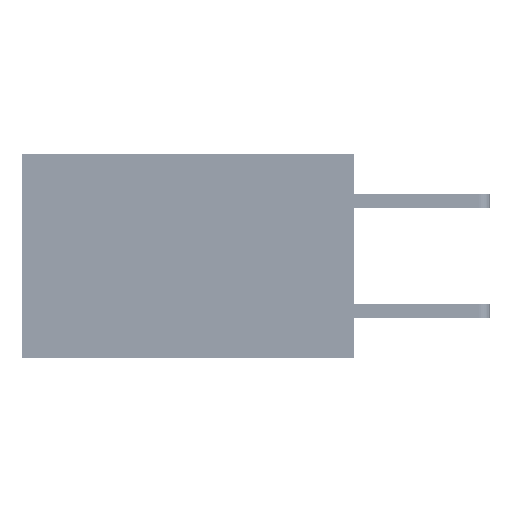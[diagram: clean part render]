
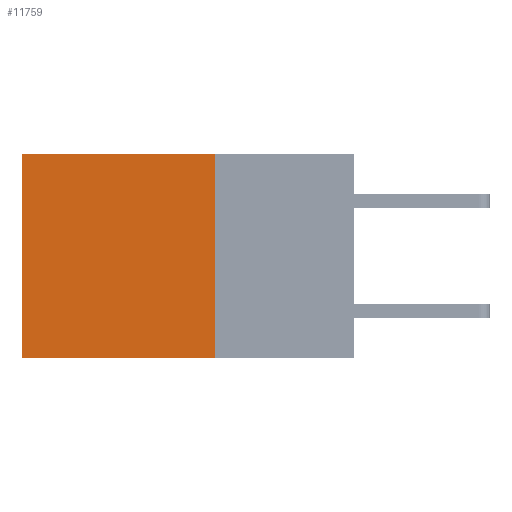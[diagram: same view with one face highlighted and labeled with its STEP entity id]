
A CAD part, left-side view. The second image highlights one B-rep face of the part: STEP entity #11759.
In plain terms, the highlighted planar face has unit normal (-1, 0, 0).
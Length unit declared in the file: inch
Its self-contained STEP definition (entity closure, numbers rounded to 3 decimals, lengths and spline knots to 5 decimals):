
#631 = DIRECTION ( 'NONE',  ( 0., 0., -1. ) ) ;
#2991 = VERTEX_POINT ( 'NONE', #26524 ) ;
#5545 = PLANE ( 'NONE',  #13367 ) ;
#6780 = LINE ( 'NONE', #41627, #39125 ) ;
#8586 = DIRECTION ( 'NONE',  ( 0., 0., -1. ) ) ;
#9468 = EDGE_CURVE ( 'NONE', #12909, #18401, #6780, .T. ) ;
#11207 = CARTESIAN_POINT ( 'NONE',  ( 0.2875, 0.25, 0. ) ) ;
#11418 = LINE ( 'NONE', #24090, #28578 ) ;
#11658 = CARTESIAN_POINT ( 'NONE',  ( 0.2875, 0.25, 0. ) ) ;
#11759 = ADVANCED_FACE ( 'NONE', ( #35280 ), #5545, .F. ) ;
#12386 = EDGE_LOOP ( 'NONE', ( #23890, #41944, #21799, #23471 ) ) ;
#12909 = VERTEX_POINT ( 'NONE', #42893 ) ;
#13367 = AXIS2_PLACEMENT_3D ( 'NONE', #28836, #28555, #8586 ) ;
#13528 = VECTOR ( 'NONE', #28085, 39.37008 ) ;
#18401 = VERTEX_POINT ( 'NONE', #35688 ) ;
#19248 = CARTESIAN_POINT ( 'NONE',  ( 0.2875, 0.25, 0. ) ) ;
#19585 = EDGE_CURVE ( 'NONE', #2991, #18401, #11418, .T. ) ;
#21799 = ORIENTED_EDGE ( 'NONE', *, *, #22409, .F. ) ;
#22409 = EDGE_CURVE ( 'NONE', #29419, #2991, #37310, .T. ) ;
#23471 = ORIENTED_EDGE ( 'NONE', *, *, #37540, .T. ) ;
#23890 = ORIENTED_EDGE ( 'NONE', *, *, #9468, .T. ) ;
#24090 = CARTESIAN_POINT ( 'NONE',  ( 0.2875, 0.25, -0.37 ) ) ;
#24665 = DIRECTION ( 'NONE',  ( 0., 0., -1. ) ) ;
#26524 = CARTESIAN_POINT ( 'NONE',  ( 0.2875, 0.25, -0.37 ) ) ;
#26531 = LINE ( 'NONE', #11658, #13528 ) ;
#28085 = DIRECTION ( 'NONE',  ( 0., 1., 0. ) ) ;
#28555 = DIRECTION ( 'NONE',  ( 1., 0., 0. ) ) ;
#28578 = VECTOR ( 'NONE', #30349, 39.37008 ) ;
#28836 = CARTESIAN_POINT ( 'NONE',  ( 0.2875, 0.25, 0. ) ) ;
#29419 = VERTEX_POINT ( 'NONE', #11207 ) ;
#30349 = DIRECTION ( 'NONE',  ( 0., 1., 0. ) ) ;
#35280 = FACE_OUTER_BOUND ( 'NONE', #12386, .T. ) ;
#35688 = CARTESIAN_POINT ( 'NONE',  ( 0.2875, 0.6, -0.37 ) ) ;
#37310 = LINE ( 'NONE', #19248, #39430 ) ;
#37540 = EDGE_CURVE ( 'NONE', #29419, #12909, #26531, .T. ) ;
#39125 = VECTOR ( 'NONE', #24665, 39.37008 ) ;
#39430 = VECTOR ( 'NONE', #631, 39.37008 ) ;
#41627 = CARTESIAN_POINT ( 'NONE',  ( 0.2875, 0.6, 0. ) ) ;
#41944 = ORIENTED_EDGE ( 'NONE', *, *, #19585, .F. ) ;
#42893 = CARTESIAN_POINT ( 'NONE',  ( 0.2875, 0.6, 0. ) ) ;
